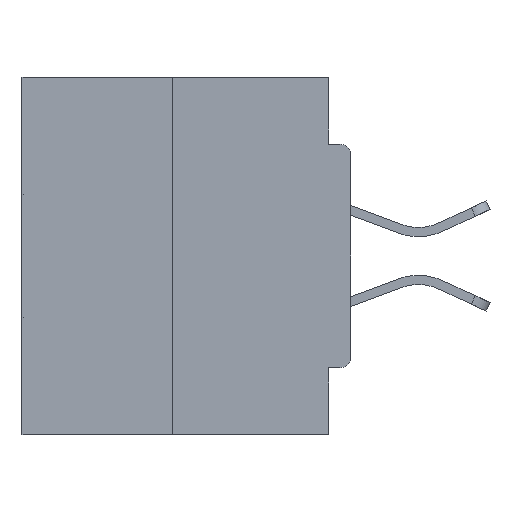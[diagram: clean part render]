
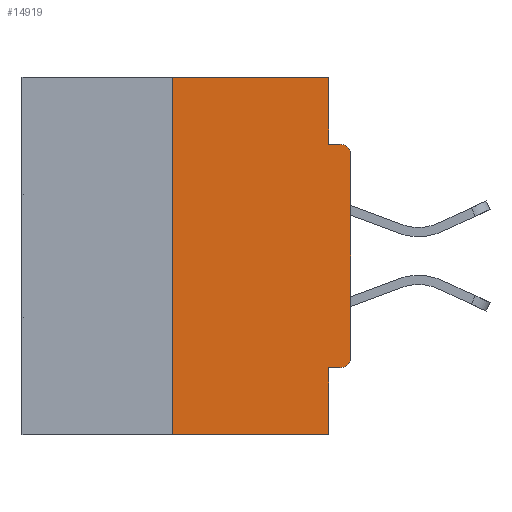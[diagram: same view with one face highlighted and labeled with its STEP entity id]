
A CAD part, left-side view. The second image highlights one B-rep face of the part: STEP entity #14919.
In plain terms, the highlighted planar face has unit normal (-1, 0, 0).
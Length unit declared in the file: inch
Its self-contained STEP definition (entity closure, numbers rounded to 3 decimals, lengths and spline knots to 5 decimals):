
#190 = EDGE_CURVE ( 'NONE', #36090, #35953, #14009, .T. ) ;
#2245 = ORIENTED_EDGE ( 'NONE', *, *, #8273, .F. ) ;
#2448 = LINE ( 'NONE', #14368, #13837 ) ;
#3070 = VECTOR ( 'NONE', #23736, 39.37008 ) ;
#3621 = VECTOR ( 'NONE', #12423, 39.37008 ) ;
#3823 = ORIENTED_EDGE ( 'NONE', *, *, #16614, .F. ) ;
#4248 = CARTESIAN_POINT ( 'NONE',  ( 0., 0.25, 0. ) ) ;
#4776 = EDGE_CURVE ( 'NONE', #32823, #24095, #27361, .T. ) ;
#5292 = EDGE_CURVE ( 'NONE', #20429, #38329, #25403, .T. ) ;
#6433 = ORIENTED_EDGE ( 'NONE', *, *, #29501, .F. ) ;
#6441 = DIRECTION ( 'NONE',  ( 0., 0., 1. ) ) ;
#6523 = LINE ( 'NONE', #21460, #26000 ) ;
#7121 = EDGE_CURVE ( 'NONE', #19018, #7207, #7651, .T. ) ;
#7207 = VERTEX_POINT ( 'NONE', #33442 ) ;
#7615 = CARTESIAN_POINT ( 'NONE',  ( 0., 0.25, -0.5 ) ) ;
#7651 = CIRCLE ( 'NONE', #35283, 0.015 ) ;
#7690 = VERTEX_POINT ( 'NONE', #23989 ) ;
#8273 = EDGE_CURVE ( 'NONE', #19018, #20429, #35488, .T. ) ;
#9309 = DIRECTION ( 'NONE',  ( 0., -1., 0. ) ) ;
#9806 = DIRECTION ( 'NONE',  ( 0., 0., -1. ) ) ;
#10658 = AXIS2_PLACEMENT_3D ( 'NONE', #16386, #13437, #16514 ) ;
#11530 = CARTESIAN_POINT ( 'NONE',  ( 0., 0.031, -0.4065 ) ) ;
#11821 = DIRECTION ( 'NONE',  ( -1., 0., 0. ) ) ;
#12423 = DIRECTION ( 'NONE',  ( 0., 0., -1. ) ) ;
#13129 = CARTESIAN_POINT ( 'NONE',  ( 0., 0.46, 0. ) ) ;
#13211 = CARTESIAN_POINT ( 'NONE',  ( 0., 0., -0.4065 ) ) ;
#13437 = DIRECTION ( 'NONE',  ( -1., 0., 0. ) ) ;
#13837 = VECTOR ( 'NONE', #35578, 39.37008 ) ;
#14009 = CIRCLE ( 'NONE', #10658, 0.015 ) ;
#14322 = ORIENTED_EDGE ( 'NONE', *, *, #22609, .T. ) ;
#14327 = DIRECTION ( 'NONE',  ( 0., 0., 1. ) ) ;
#14368 = CARTESIAN_POINT ( 'NONE',  ( 0., 0.46, 0. ) ) ;
#14892 = AXIS2_PLACEMENT_3D ( 'NONE', #13129, #16191, #9806 ) ;
#14913 = CARTESIAN_POINT ( 'NONE',  ( 0., 0.031, -0.5 ) ) ;
#14919 = ADVANCED_FACE ( 'NONE', ( #37882 ), #34357, .F. ) ;
#16191 = DIRECTION ( 'NONE',  ( 1., 0., 0. ) ) ;
#16276 = DIRECTION ( 'NONE',  ( 0., 1., 0. ) ) ;
#16386 = CARTESIAN_POINT ( 'NONE',  ( 0., 0.015, -0.1085 ) ) ;
#16514 = DIRECTION ( 'NONE',  ( 0., 0., -1. ) ) ;
#16614 = EDGE_CURVE ( 'NONE', #23076, #7690, #31076, .T. ) ;
#17668 = CARTESIAN_POINT ( 'NONE',  ( 0., 0.015, -0.3915 ) ) ;
#19018 = VERTEX_POINT ( 'NONE', #28444 ) ;
#19945 = ORIENTED_EDGE ( 'NONE', *, *, #4776, .F. ) ;
#20429 = VERTEX_POINT ( 'NONE', #11530 ) ;
#21137 = DIRECTION ( 'NONE',  ( 0., 0., -1. ) ) ;
#21240 = EDGE_CURVE ( 'NONE', #24095, #35953, #35342, .T. ) ;
#21256 = ORIENTED_EDGE ( 'NONE', *, *, #190, .T. ) ;
#21460 = CARTESIAN_POINT ( 'NONE',  ( 0., 0., 0. ) ) ;
#21615 = ORIENTED_EDGE ( 'NONE', *, *, #7121, .T. ) ;
#21971 = CARTESIAN_POINT ( 'NONE',  ( 0., 0.015, -0.0935 ) ) ;
#22609 = EDGE_CURVE ( 'NONE', #23076, #38329, #34308, .T. ) ;
#23076 = VERTEX_POINT ( 'NONE', #7615 ) ;
#23736 = DIRECTION ( 'NONE',  ( 0., -1., 0. ) ) ;
#23989 = CARTESIAN_POINT ( 'NONE',  ( 0., 0.25, 0. ) ) ;
#24095 = VERTEX_POINT ( 'NONE', #32901 ) ;
#24630 = EDGE_CURVE ( 'NONE', #7207, #36090, #6523, .T. ) ;
#25403 = LINE ( 'NONE', #39317, #38267 ) ;
#25957 = ORIENTED_EDGE ( 'NONE', *, *, #5292, .F. ) ;
#26000 = VECTOR ( 'NONE', #6441, 39.37008 ) ;
#26183 = VECTOR ( 'NONE', #9309, 39.37008 ) ;
#27361 = LINE ( 'NONE', #33660, #3621 ) ;
#28444 = CARTESIAN_POINT ( 'NONE',  ( 0., 0.015, -0.4065 ) ) ;
#29501 = EDGE_CURVE ( 'NONE', #7690, #32823, #2448, .T. ) ;
#29742 = CARTESIAN_POINT ( 'NONE',  ( 0., 0., -0.1085 ) ) ;
#29885 = CARTESIAN_POINT ( 'NONE',  ( 0., 0.46, -0.5 ) ) ;
#31076 = LINE ( 'NONE', #4248, #32509 ) ;
#32509 = VECTOR ( 'NONE', #14327, 39.37008 ) ;
#32778 = CARTESIAN_POINT ( 'NONE',  ( 0., 0.031, 0. ) ) ;
#32823 = VERTEX_POINT ( 'NONE', #32778 ) ;
#32901 = CARTESIAN_POINT ( 'NONE',  ( 0., 0.031, -0.0935 ) ) ;
#33442 = CARTESIAN_POINT ( 'NONE',  ( 0., 0., -0.3915 ) ) ;
#33660 = CARTESIAN_POINT ( 'NONE',  ( 0., 0.031, 0. ) ) ;
#34308 = LINE ( 'NONE', #29885, #26183 ) ;
#34357 = PLANE ( 'NONE',  #14892 ) ;
#34789 = ORIENTED_EDGE ( 'NONE', *, *, #21240, .F. ) ;
#35283 = AXIS2_PLACEMENT_3D ( 'NONE', #17668, #11821, #38893 ) ;
#35311 = EDGE_LOOP ( 'NONE', ( #6433, #3823, #14322, #25957, #2245, #21615, #38843, #21256, #34789, #19945 ) ) ;
#35342 = LINE ( 'NONE', #36228, #3070 ) ;
#35488 = LINE ( 'NONE', #13211, #35999 ) ;
#35578 = DIRECTION ( 'NONE',  ( 0., -1., 0. ) ) ;
#35953 = VERTEX_POINT ( 'NONE', #21971 ) ;
#35999 = VECTOR ( 'NONE', #16276, 39.37008 ) ;
#36090 = VERTEX_POINT ( 'NONE', #29742 ) ;
#36228 = CARTESIAN_POINT ( 'NONE',  ( 0., 0., -0.0935 ) ) ;
#37882 = FACE_OUTER_BOUND ( 'NONE', #35311, .T. ) ;
#38267 = VECTOR ( 'NONE', #21137, 39.37008 ) ;
#38329 = VERTEX_POINT ( 'NONE', #14913 ) ;
#38843 = ORIENTED_EDGE ( 'NONE', *, *, #24630, .T. ) ;
#38893 = DIRECTION ( 'NONE',  ( 0., 0., -1. ) ) ;
#39317 = CARTESIAN_POINT ( 'NONE',  ( 0., 0.031, -0.5 ) ) ;
